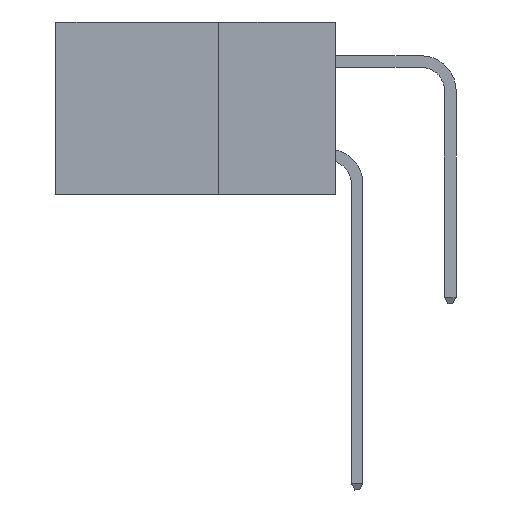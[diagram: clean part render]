
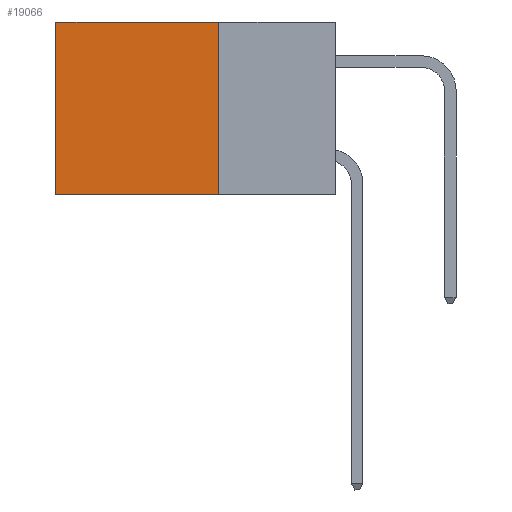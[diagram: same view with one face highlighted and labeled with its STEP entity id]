
A CAD part, left-side view. The second image highlights one B-rep face of the part: STEP entity #19066.
In plain terms, the highlighted planar face has unit normal (-1, 0, 0).
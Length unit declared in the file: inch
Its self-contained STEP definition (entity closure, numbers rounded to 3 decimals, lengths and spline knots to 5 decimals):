
#3162 = CARTESIAN_POINT ( 'NONE',  ( 0.2875, 0.6, -0.37 ) ) ;
#3434 = AXIS2_PLACEMENT_3D ( 'NONE', #41847, #41416, #17607 ) ;
#3522 = VERTEX_POINT ( 'NONE', #35779 ) ;
#3760 = PLANE ( 'NONE',  #3434 ) ;
#7267 = LINE ( 'NONE', #41290, #8850 ) ;
#8161 = VECTOR ( 'NONE', #23785, 39.37008 ) ;
#8850 = VECTOR ( 'NONE', #13871, 39.37008 ) ;
#9498 = DIRECTION ( 'NONE',  ( 0., 0., -1. ) ) ;
#11568 = ORIENTED_EDGE ( 'NONE', *, *, #28644, .T. ) ;
#12219 = CARTESIAN_POINT ( 'NONE',  ( 0.2875, 0.25, 0. ) ) ;
#12344 = CARTESIAN_POINT ( 'NONE',  ( 0.2875, 0.6, 0. ) ) ;
#13345 = LINE ( 'NONE', #37163, #8161 ) ;
#13871 = DIRECTION ( 'NONE',  ( 0., 1., 0. ) ) ;
#15426 = VERTEX_POINT ( 'NONE', #17243 ) ;
#16777 = EDGE_CURVE ( 'NONE', #3522, #39690, #7267, .T. ) ;
#17243 = CARTESIAN_POINT ( 'NONE',  ( 0.2875, 0.6, 0. ) ) ;
#17607 = DIRECTION ( 'NONE',  ( 0., 0., -1. ) ) ;
#19066 = ADVANCED_FACE ( 'NONE', ( #23764 ), #3760, .F. ) ;
#20559 = EDGE_LOOP ( 'NONE', ( #38213, #38707, #25053, #11568 ) ) ;
#23531 = EDGE_CURVE ( 'NONE', #15426, #39690, #29342, .T. ) ;
#23764 = FACE_OUTER_BOUND ( 'NONE', #20559, .T. ) ;
#23785 = DIRECTION ( 'NONE',  ( 0., 1., 0. ) ) ;
#25053 = ORIENTED_EDGE ( 'NONE', *, *, #29797, .F. ) ;
#28508 = VECTOR ( 'NONE', #9498, 39.37008 ) ;
#28644 = EDGE_CURVE ( 'NONE', #29755, #15426, #13345, .T. ) ;
#29342 = LINE ( 'NONE', #12344, #44202 ) ;
#29755 = VERTEX_POINT ( 'NONE', #41910 ) ;
#29797 = EDGE_CURVE ( 'NONE', #29755, #3522, #36461, .T. ) ;
#35779 = CARTESIAN_POINT ( 'NONE',  ( 0.2875, 0.25, -0.37 ) ) ;
#36461 = LINE ( 'NONE', #12219, #28508 ) ;
#37163 = CARTESIAN_POINT ( 'NONE',  ( 0.2875, 0.25, 0. ) ) ;
#38213 = ORIENTED_EDGE ( 'NONE', *, *, #23531, .T. ) ;
#38707 = ORIENTED_EDGE ( 'NONE', *, *, #16777, .F. ) ;
#39690 = VERTEX_POINT ( 'NONE', #3162 ) ;
#41290 = CARTESIAN_POINT ( 'NONE',  ( 0.2875, 0.25, -0.37 ) ) ;
#41416 = DIRECTION ( 'NONE',  ( 1., 0., 0. ) ) ;
#41847 = CARTESIAN_POINT ( 'NONE',  ( 0.2875, 0.25, 0. ) ) ;
#41910 = CARTESIAN_POINT ( 'NONE',  ( 0.2875, 0.25, 0. ) ) ;
#43159 = DIRECTION ( 'NONE',  ( 0., 0., -1. ) ) ;
#44202 = VECTOR ( 'NONE', #43159, 39.37008 ) ;
